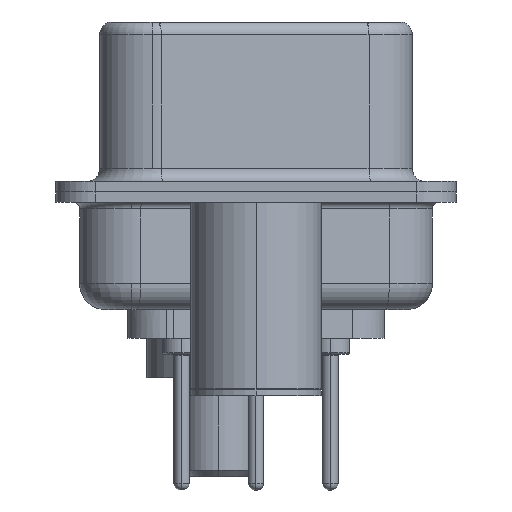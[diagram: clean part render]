
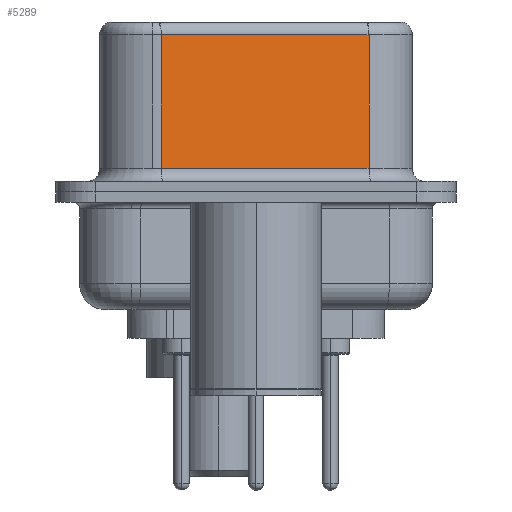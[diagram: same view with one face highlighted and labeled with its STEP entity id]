
A CAD part, left-side view. The second image highlights one B-rep face of the part: STEP entity #5289.
In plain terms, the highlighted planar face has unit normal (-0.985, -0.174, 0).
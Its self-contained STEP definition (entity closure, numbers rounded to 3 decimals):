
#1375 = ORIENTED_EDGE ( 'NONE', *, *, #1384, .T. ) ;
#1384 = EDGE_CURVE ( 'NONE', #24707, #18133, #17249, .T. ) ;
#2019 = DIRECTION ( 'NONE',  ( 0., 0., -1. ) ) ;
#2305 = DIRECTION ( 'NONE',  ( 0., 0., -1. ) ) ;
#4318 = CARTESIAN_POINT ( 'NONE',  ( 5.132, -4.322, 0.9 ) ) ;
#4429 = EDGE_CURVE ( 'NONE', #24006, #25307, #15248, .T. ) ;
#5027 = CARTESIAN_POINT ( 'NONE',  ( 5.132, -4.322, 0.9 ) ) ;
#5289 = ADVANCED_FACE ( 'NONE', ( #19921 ), #21798, .F. ) ;
#5382 = AXIS2_PLACEMENT_3D ( 'NONE', #14757, #12552, #24232 ) ;
#5960 = EDGE_CURVE ( 'NONE', #24006, #24707, #16653, .T. ) ;
#7199 = VECTOR ( 'NONE', #14317, 1000. ) ;
#7229 = CARTESIAN_POINT ( 'NONE',  ( 5.132, -4.322, 6.02 ) ) ;
#7350 = ORIENTED_EDGE ( 'NONE', *, *, #12035, .T. ) ;
#9578 = DIRECTION ( 'NONE',  ( 0.174, -0.985, 0. ) ) ;
#10005 = EDGE_LOOP ( 'NONE', ( #11184, #18920, #1375, #7350 ) ) ;
#11184 = ORIENTED_EDGE ( 'NONE', *, *, #4429, .F. ) ;
#11668 = CARTESIAN_POINT ( 'NONE',  ( 3.73, 3.628, 6.52 ) ) ;
#11723 = VECTOR ( 'NONE', #9578, 1000. ) ;
#12035 = EDGE_CURVE ( 'NONE', #18133, #25307, #18248, .T. ) ;
#12552 = DIRECTION ( 'NONE',  ( 0.985, 0.174, 0. ) ) ;
#13165 = CARTESIAN_POINT ( 'NONE',  ( 5.132, -4.322, 6.52 ) ) ;
#14317 = DIRECTION ( 'NONE',  ( -0.174, 0.985, 0. ) ) ;
#14757 = CARTESIAN_POINT ( 'NONE',  ( 5.132, -4.322, 6.52 ) ) ;
#15248 = LINE ( 'NONE', #13165, #16737 ) ;
#16653 = LINE ( 'NONE', #7229, #7199 ) ;
#16737 = VECTOR ( 'NONE', #2019, 1000. ) ;
#17249 = LINE ( 'NONE', #11668, #27828 ) ;
#17895 = CARTESIAN_POINT ( 'NONE',  ( 3.73, 3.628, 0.9 ) ) ;
#18133 = VERTEX_POINT ( 'NONE', #17895 ) ;
#18248 = LINE ( 'NONE', #5027, #11723 ) ;
#18920 = ORIENTED_EDGE ( 'NONE', *, *, #5960, .T. ) ;
#19921 = FACE_OUTER_BOUND ( 'NONE', #10005, .T. ) ;
#21798 = PLANE ( 'NONE',  #5382 ) ;
#24006 = VERTEX_POINT ( 'NONE', #25650 ) ;
#24232 = DIRECTION ( 'NONE',  ( -0.174, 0.985, 0. ) ) ;
#24707 = VERTEX_POINT ( 'NONE', #28322 ) ;
#25307 = VERTEX_POINT ( 'NONE', #4318 ) ;
#25650 = CARTESIAN_POINT ( 'NONE',  ( 5.132, -4.322, 6.02 ) ) ;
#27828 = VECTOR ( 'NONE', #2305, 1000. ) ;
#28322 = CARTESIAN_POINT ( 'NONE',  ( 3.73, 3.628, 6.02 ) ) ;
